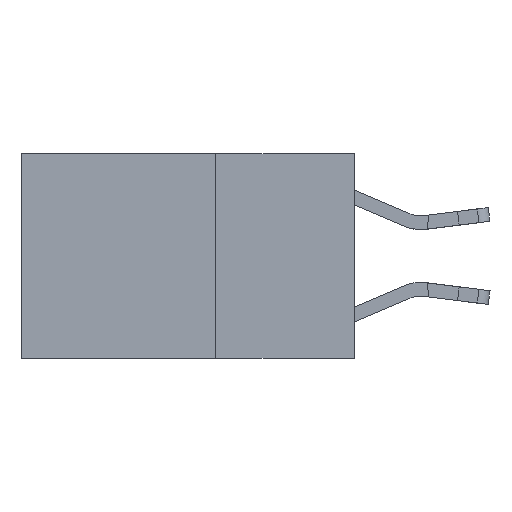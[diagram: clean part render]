
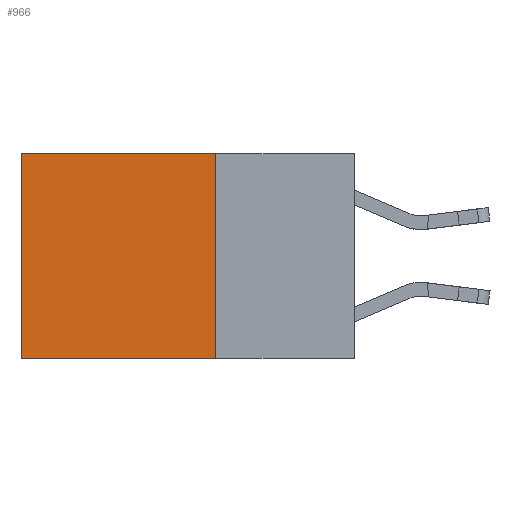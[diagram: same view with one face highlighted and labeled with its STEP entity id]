
A CAD part, left-side view. The second image highlights one B-rep face of the part: STEP entity #966.
In plain terms, the highlighted planar face has unit normal (-1, 0, 0).
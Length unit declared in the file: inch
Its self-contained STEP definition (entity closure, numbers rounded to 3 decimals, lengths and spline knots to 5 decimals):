
#37 = PLANE ( 'NONE',  #1156 ) ;
#372 = FACE_OUTER_BOUND ( 'NONE', #13272, .T. ) ;
#966 = ADVANCED_FACE ( 'NONE', ( #372 ), #37, .F. ) ;
#1156 = AXIS2_PLACEMENT_3D ( 'NONE', #14421, #1753, #13012 ) ;
#1753 = DIRECTION ( 'NONE',  ( 1., 0., 0. ) ) ;
#3803 = ORIENTED_EDGE ( 'NONE', *, *, #19896, .T. ) ;
#4353 = ORIENTED_EDGE ( 'NONE', *, *, #14392, .F. ) ;
#5437 = DIRECTION ( 'NONE',  ( 0., 1., 0. ) ) ;
#5553 = VERTEX_POINT ( 'NONE', #16970 ) ;
#6463 = VECTOR ( 'NONE', #5437, 39.37008 ) ;
#6856 = DIRECTION ( 'NONE',  ( 0., 0., -1. ) ) ;
#8079 = ORIENTED_EDGE ( 'NONE', *, *, #9698, .F. ) ;
#8333 = CARTESIAN_POINT ( 'NONE',  ( 0.2625, 0.25, -0.37 ) ) ;
#8572 = ORIENTED_EDGE ( 'NONE', *, *, #18390, .T. ) ;
#8826 = CARTESIAN_POINT ( 'NONE',  ( 0.2625, 0.25, -0.37 ) ) ;
#9698 = EDGE_CURVE ( 'NONE', #17725, #13691, #16251, .T. ) ;
#9972 = CARTESIAN_POINT ( 'NONE',  ( 0.2625, 0.6, 0. ) ) ;
#10191 = VECTOR ( 'NONE', #6856, 39.37008 ) ;
#10331 = VECTOR ( 'NONE', #17730, 39.37008 ) ;
#10681 = LINE ( 'NONE', #19150, #10191 ) ;
#11105 = LINE ( 'NONE', #13253, #6463 ) ;
#13012 = DIRECTION ( 'NONE',  ( 0., 0., -1. ) ) ;
#13253 = CARTESIAN_POINT ( 'NONE',  ( 0.2625, 0.25, 0. ) ) ;
#13272 = EDGE_LOOP ( 'NONE', ( #3803, #8079, #4353, #8572 ) ) ;
#13691 = VERTEX_POINT ( 'NONE', #18609 ) ;
#14392 = EDGE_CURVE ( 'NONE', #5553, #17725, #10681, .T. ) ;
#14421 = CARTESIAN_POINT ( 'NONE',  ( 0.2625, 0.25, 0. ) ) ;
#14930 = VERTEX_POINT ( 'NONE', #15674 ) ;
#15674 = CARTESIAN_POINT ( 'NONE',  ( 0.2625, 0.6, 0. ) ) ;
#16148 = DIRECTION ( 'NONE',  ( 0., 1., 0. ) ) ;
#16251 = LINE ( 'NONE', #8333, #19319 ) ;
#16970 = CARTESIAN_POINT ( 'NONE',  ( 0.2625, 0.25, 0. ) ) ;
#17725 = VERTEX_POINT ( 'NONE', #8826 ) ;
#17730 = DIRECTION ( 'NONE',  ( 0., 0., -1. ) ) ;
#18390 = EDGE_CURVE ( 'NONE', #5553, #14930, #11105, .T. ) ;
#18609 = CARTESIAN_POINT ( 'NONE',  ( 0.2625, 0.6, -0.37 ) ) ;
#19150 = CARTESIAN_POINT ( 'NONE',  ( 0.2625, 0.25, 0. ) ) ;
#19319 = VECTOR ( 'NONE', #16148, 39.37008 ) ;
#19472 = LINE ( 'NONE', #9972, #10331 ) ;
#19896 = EDGE_CURVE ( 'NONE', #14930, #13691, #19472, .T. ) ;
